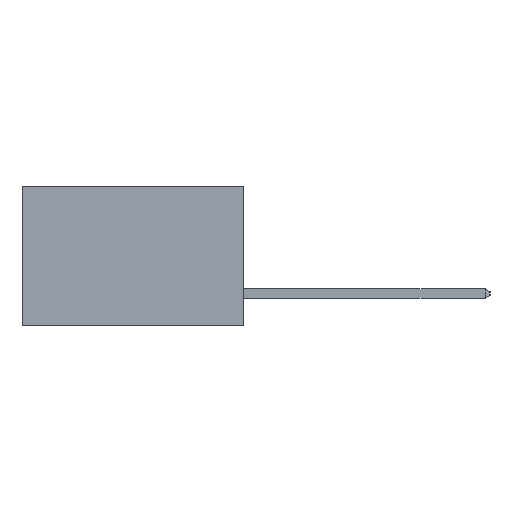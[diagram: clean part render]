
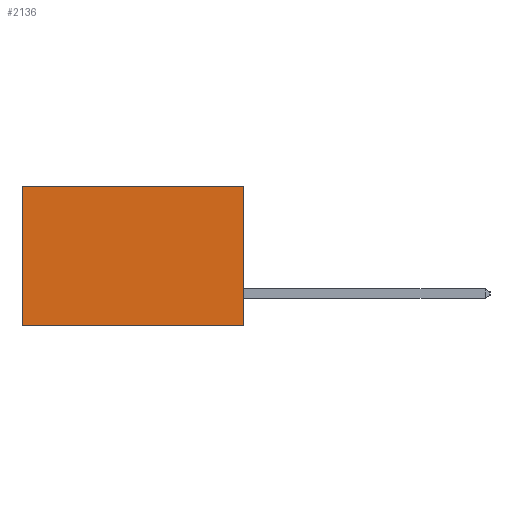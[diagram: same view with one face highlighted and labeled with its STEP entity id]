
A CAD part, left-side view. The second image highlights one B-rep face of the part: STEP entity #2136.
In plain terms, the highlighted planar face has unit normal (-1, 0, 0).
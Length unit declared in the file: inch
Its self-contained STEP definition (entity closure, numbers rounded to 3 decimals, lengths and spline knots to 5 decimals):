
#1223 = VECTOR ( 'NONE', #14773, 39.37008 ) ;
#1378 = CARTESIAN_POINT ( 'NONE',  ( 0.277, 0.59, -0.37 ) ) ;
#2136 = ADVANCED_FACE ( 'NONE', ( #17171 ), #7801, .F. ) ;
#2951 = ORIENTED_EDGE ( 'NONE', *, *, #13171, .F. ) ;
#3011 = VERTEX_POINT ( 'NONE', #3015 ) ;
#3015 = CARTESIAN_POINT ( 'NONE',  ( 0.277, 0., -0.37 ) ) ;
#4111 = DIRECTION ( 'NONE',  ( 0., 1., 0. ) ) ;
#4266 = EDGE_CURVE ( 'NONE', #15967, #9216, #6486, .T. ) ;
#4893 = DIRECTION ( 'NONE',  ( 0., 0., -1. ) ) ;
#4986 = EDGE_CURVE ( 'NONE', #9216, #5800, #17544, .T. ) ;
#5075 = EDGE_LOOP ( 'NONE', ( #19926, #2951, #12079, #9402 ) ) ;
#5800 = VERTEX_POINT ( 'NONE', #1378 ) ;
#6486 = LINE ( 'NONE', #14468, #10198 ) ;
#6969 = CARTESIAN_POINT ( 'NONE',  ( 0.277, 0., -0.37 ) ) ;
#7801 = PLANE ( 'NONE',  #16114 ) ;
#9216 = VERTEX_POINT ( 'NONE', #14995 ) ;
#9402 = ORIENTED_EDGE ( 'NONE', *, *, #4266, .T. ) ;
#9601 = CARTESIAN_POINT ( 'NONE',  ( 0.277, 0., -0.37 ) ) ;
#9669 = VECTOR ( 'NONE', #4893, 39.37008 ) ;
#9717 = DIRECTION ( 'NONE',  ( 0., 0., -1. ) ) ;
#10085 = CARTESIAN_POINT ( 'NONE',  ( 0.277, 0., 0. ) ) ;
#10198 = VECTOR ( 'NONE', #14272, 39.37008 ) ;
#12079 = ORIENTED_EDGE ( 'NONE', *, *, #18227, .F. ) ;
#13171 = EDGE_CURVE ( 'NONE', #3011, #5800, #19220, .T. ) ;
#13567 = CARTESIAN_POINT ( 'NONE',  ( 0.277, 0., -0.37 ) ) ;
#13824 = DIRECTION ( 'NONE',  ( 1., 0., 0. ) ) ;
#13845 = LINE ( 'NONE', #9601, #9669 ) ;
#14272 = DIRECTION ( 'NONE',  ( 0., 1., 0. ) ) ;
#14468 = CARTESIAN_POINT ( 'NONE',  ( 0.277, 0., 0. ) ) ;
#14773 = DIRECTION ( 'NONE',  ( 0., 0., -1. ) ) ;
#14840 = CARTESIAN_POINT ( 'NONE',  ( 0.277, 0.59, -0.37 ) ) ;
#14995 = CARTESIAN_POINT ( 'NONE',  ( 0.277, 0.59, 0. ) ) ;
#15064 = VECTOR ( 'NONE', #4111, 39.37008 ) ;
#15967 = VERTEX_POINT ( 'NONE', #10085 ) ;
#16114 = AXIS2_PLACEMENT_3D ( 'NONE', #6969, #13824, #9717 ) ;
#17171 = FACE_OUTER_BOUND ( 'NONE', #5075, .T. ) ;
#17544 = LINE ( 'NONE', #14840, #1223 ) ;
#18227 = EDGE_CURVE ( 'NONE', #15967, #3011, #13845, .T. ) ;
#19220 = LINE ( 'NONE', #13567, #15064 ) ;
#19926 = ORIENTED_EDGE ( 'NONE', *, *, #4986, .T. ) ;
